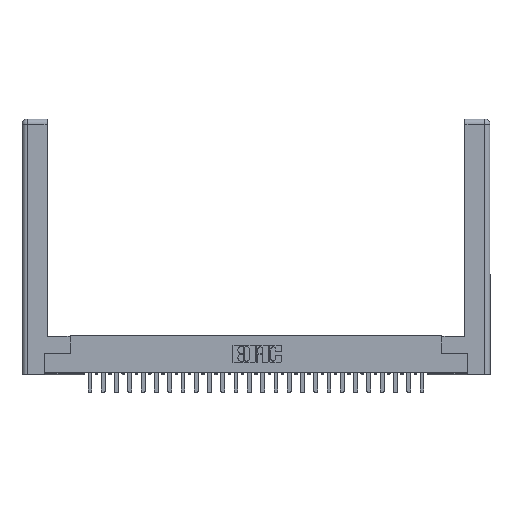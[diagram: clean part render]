
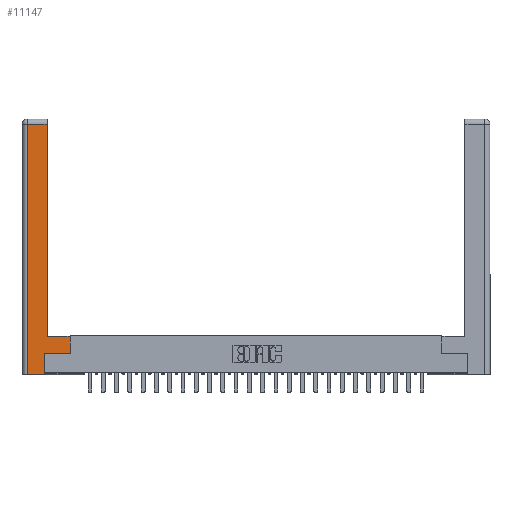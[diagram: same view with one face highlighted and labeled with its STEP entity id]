
A CAD part, top view. The second image highlights one B-rep face of the part: STEP entity #11147.
In plain terms, the highlighted planar face has unit normal (0, 0, 1).
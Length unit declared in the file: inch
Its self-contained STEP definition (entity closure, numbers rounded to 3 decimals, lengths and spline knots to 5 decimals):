
#1037 = CARTESIAN_POINT ( 'NONE',  ( 0.295, 3., 0. ) ) ;
#1356 = VECTOR ( 'NONE', #3649, 39.37008 ) ;
#1574 = VERTEX_POINT ( 'NONE', #18879 ) ;
#1634 = ORIENTED_EDGE ( 'NONE', *, *, #13628, .T. ) ;
#2102 = CARTESIAN_POINT ( 'NONE',  ( 0.265, 0., 0. ) ) ;
#2270 = VECTOR ( 'NONE', #5885, 39.37008 ) ;
#2277 = EDGE_CURVE ( 'NONE', #2928, #7460, #30344, .T. ) ;
#2416 = DIRECTION ( 'NONE',  ( 0., -1., 0. ) ) ;
#2928 = VERTEX_POINT ( 'NONE', #2102 ) ;
#3410 = ORIENTED_EDGE ( 'NONE', *, *, #24564, .T. ) ;
#3544 = CARTESIAN_POINT ( 'NONE',  ( 0.265, 0.245, 0. ) ) ;
#3570 = ORIENTED_EDGE ( 'NONE', *, *, #2277, .T. ) ;
#3649 = DIRECTION ( 'NONE',  ( -1., 0., 0. ) ) ;
#3745 = DIRECTION ( 'NONE',  ( -1., 0., 0. ) ) ;
#3802 = VERTEX_POINT ( 'NONE', #26759 ) ;
#3855 = LINE ( 'NONE', #1037, #2270 ) ;
#4664 = DIRECTION ( 'NONE',  ( -1., 0., 0. ) ) ;
#4729 = CARTESIAN_POINT ( 'NONE',  ( 0.265, 0., 0. ) ) ;
#4913 = EDGE_CURVE ( 'NONE', #3802, #23425, #24051, .T. ) ;
#5057 = EDGE_CURVE ( 'NONE', #23734, #16481, #22894, .T. ) ;
#5469 = CARTESIAN_POINT ( 'NONE',  ( 0.265, 0.245, 0. ) ) ;
#5515 = LINE ( 'NONE', #5585, #23646 ) ;
#5585 = CARTESIAN_POINT ( 'NONE',  ( 0.565, 0.45, 0. ) ) ;
#5885 = DIRECTION ( 'NONE',  ( 0., 1., 0. ) ) ;
#6343 = VECTOR ( 'NONE', #2416, 39.37008 ) ;
#6985 = DIRECTION ( 'NONE',  ( 0., 0., -1. ) ) ;
#7120 = LINE ( 'NONE', #4729, #25615 ) ;
#7167 = CARTESIAN_POINT ( 'NONE',  ( 0.0615, 0., 0. ) ) ;
#7243 = LINE ( 'NONE', #21015, #1356 ) ;
#7460 = VERTEX_POINT ( 'NONE', #3544 ) ;
#7907 = DIRECTION ( 'NONE',  ( 0., 1., 0. ) ) ;
#8634 = ORIENTED_EDGE ( 'NONE', *, *, #18261, .T. ) ;
#9364 = AXIS2_PLACEMENT_3D ( 'NONE', #27308, #6985, #4664 ) ;
#9887 = CARTESIAN_POINT ( 'NONE',  ( 0.0615, 0., 0. ) ) ;
#10702 = ORIENTED_EDGE ( 'NONE', *, *, #4913, .T. ) ;
#11147 = ADVANCED_FACE ( 'NONE', ( #18051 ), #14448, .F. ) ;
#12275 = ORIENTED_EDGE ( 'NONE', *, *, #21834, .T. ) ;
#13089 = ORIENTED_EDGE ( 'NONE', *, *, #21086, .T. ) ;
#13318 = DIRECTION ( 'NONE',  ( 1., 0., 0. ) ) ;
#13628 = EDGE_CURVE ( 'NONE', #23425, #32569, #3855, .T. ) ;
#13846 = CARTESIAN_POINT ( 'NONE',  ( 0.295, 0.45, 0. ) ) ;
#14448 = PLANE ( 'NONE',  #9364 ) ;
#15232 = DIRECTION ( 'NONE',  ( 0., 1., 0. ) ) ;
#15344 = VECTOR ( 'NONE', #3745, 39.37008 ) ;
#15837 = EDGE_LOOP ( 'NONE', ( #1634, #8634, #32511, #3410, #3570, #13089, #12275, #10702 ) ) ;
#16481 = VERTEX_POINT ( 'NONE', #7167 ) ;
#17443 = CARTESIAN_POINT ( 'NONE',  ( 0.295, 0.45, 0. ) ) ;
#17859 = LINE ( 'NONE', #23774, #21821 ) ;
#18051 = FACE_OUTER_BOUND ( 'NONE', #15837, .T. ) ;
#18261 = EDGE_CURVE ( 'NONE', #32569, #23734, #7243, .T. ) ;
#18879 = CARTESIAN_POINT ( 'NONE',  ( 0.565, 0.245, 0. ) ) ;
#21015 = CARTESIAN_POINT ( 'NONE',  ( 0.0615, 2.94, 0. ) ) ;
#21086 = EDGE_CURVE ( 'NONE', #7460, #1574, #17859, .T. ) ;
#21821 = VECTOR ( 'NONE', #13318, 39.37008 ) ;
#21834 = EDGE_CURVE ( 'NONE', #1574, #3802, #5515, .T. ) ;
#22894 = LINE ( 'NONE', #9887, #6343 ) ;
#23425 = VERTEX_POINT ( 'NONE', #17443 ) ;
#23646 = VECTOR ( 'NONE', #7907, 39.37008 ) ;
#23734 = VERTEX_POINT ( 'NONE', #27294 ) ;
#23774 = CARTESIAN_POINT ( 'NONE',  ( 0.565, 0.245, 0. ) ) ;
#24051 = LINE ( 'NONE', #13846, #15344 ) ;
#24086 = VECTOR ( 'NONE', #15232, 39.37008 ) ;
#24564 = EDGE_CURVE ( 'NONE', #16481, #2928, #7120, .T. ) ;
#25615 = VECTOR ( 'NONE', #32446, 39.37008 ) ;
#26759 = CARTESIAN_POINT ( 'NONE',  ( 0.565, 0.45, 0. ) ) ;
#27294 = CARTESIAN_POINT ( 'NONE',  ( 0.0615, 2.94, 0. ) ) ;
#27308 = CARTESIAN_POINT ( 'NONE',  ( 0., 0., 0. ) ) ;
#30344 = LINE ( 'NONE', #5469, #24086 ) ;
#30969 = CARTESIAN_POINT ( 'NONE',  ( 0.295, 2.94, 0. ) ) ;
#32446 = DIRECTION ( 'NONE',  ( 1., 0., 0. ) ) ;
#32511 = ORIENTED_EDGE ( 'NONE', *, *, #5057, .T. ) ;
#32569 = VERTEX_POINT ( 'NONE', #30969 ) ;
